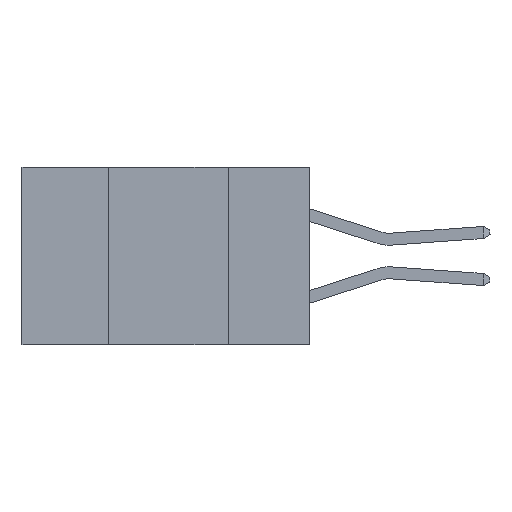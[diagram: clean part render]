
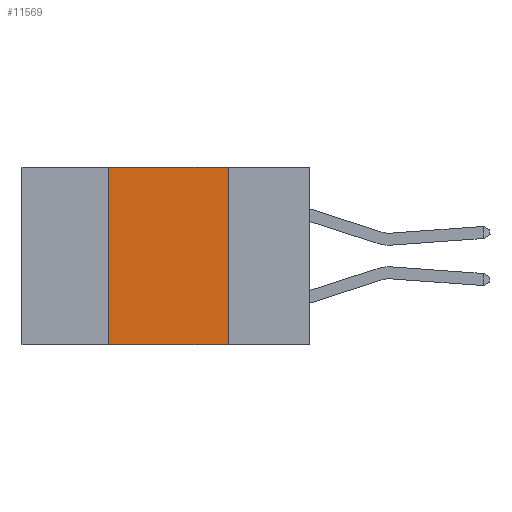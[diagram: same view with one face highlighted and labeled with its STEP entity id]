
A CAD part, left-side view. The second image highlights one B-rep face of the part: STEP entity #11569.
In plain terms, the highlighted planar face has unit normal (-1, 0, 0).
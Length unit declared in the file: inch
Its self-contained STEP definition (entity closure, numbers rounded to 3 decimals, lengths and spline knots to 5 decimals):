
#96 = ORIENTED_EDGE ( 'NONE', *, *, #4478, .F. ) ;
#165 = CARTESIAN_POINT ( 'NONE',  ( 0., 0.17, -0.37 ) ) ;
#1410 = LINE ( 'NONE', #9812, #3925 ) ;
#1760 = PLANE ( 'NONE',  #5299 ) ;
#1790 = VERTEX_POINT ( 'NONE', #10025 ) ;
#1830 = VECTOR ( 'NONE', #5807, 39.37008 ) ;
#1998 = VECTOR ( 'NONE', #4854, 39.37008 ) ;
#2380 = VERTEX_POINT ( 'NONE', #11120 ) ;
#3196 = EDGE_CURVE ( 'NONE', #1790, #10162, #1410, .T. ) ;
#3392 = ORIENTED_EDGE ( 'NONE', *, *, #6930, .F. ) ;
#3659 = DIRECTION ( 'NONE',  ( 1., 0., 0. ) ) ;
#3826 = EDGE_CURVE ( 'NONE', #1790, #2380, #4532, .T. ) ;
#3925 = VECTOR ( 'NONE', #9956, 39.37008 ) ;
#4478 = EDGE_CURVE ( 'NONE', #2380, #6053, #4930, .T. ) ;
#4532 = LINE ( 'NONE', #4841, #1998 ) ;
#4841 = CARTESIAN_POINT ( 'NONE',  ( 0., 0.42, -0.37 ) ) ;
#4854 = DIRECTION ( 'NONE',  ( 0., 0., 1. ) ) ;
#4930 = LINE ( 'NONE', #6743, #1830 ) ;
#5299 = AXIS2_PLACEMENT_3D ( 'NONE', #6426, #3659, #10152 ) ;
#5807 = DIRECTION ( 'NONE',  ( 0., -1., 0. ) ) ;
#6053 = VERTEX_POINT ( 'NONE', #11933 ) ;
#6426 = CARTESIAN_POINT ( 'NONE',  ( 0., 0.6, 0. ) ) ;
#6636 = FACE_OUTER_BOUND ( 'NONE', #7330, .T. ) ;
#6743 = CARTESIAN_POINT ( 'NONE',  ( 0., 0.6, 0. ) ) ;
#6930 = EDGE_CURVE ( 'NONE', #6053, #10162, #9798, .T. ) ;
#7330 = EDGE_LOOP ( 'NONE', ( #3392, #96, #8150, #9254 ) ) ;
#7567 = DIRECTION ( 'NONE',  ( 0., 0., -1. ) ) ;
#8150 = ORIENTED_EDGE ( 'NONE', *, *, #3826, .F. ) ;
#8582 = CARTESIAN_POINT ( 'NONE',  ( 0., 0.17, -0.37 ) ) ;
#9254 = ORIENTED_EDGE ( 'NONE', *, *, #3196, .T. ) ;
#9798 = LINE ( 'NONE', #165, #11911 ) ;
#9812 = CARTESIAN_POINT ( 'NONE',  ( 0., 0.6, -0.37 ) ) ;
#9956 = DIRECTION ( 'NONE',  ( 0., -1., 0. ) ) ;
#10025 = CARTESIAN_POINT ( 'NONE',  ( 0., 0.42, -0.37 ) ) ;
#10152 = DIRECTION ( 'NONE',  ( 0., 0., -1. ) ) ;
#10162 = VERTEX_POINT ( 'NONE', #8582 ) ;
#11120 = CARTESIAN_POINT ( 'NONE',  ( 0., 0.42, 0. ) ) ;
#11569 = ADVANCED_FACE ( 'NONE', ( #6636 ), #1760, .F. ) ;
#11911 = VECTOR ( 'NONE', #7567, 39.37008 ) ;
#11933 = CARTESIAN_POINT ( 'NONE',  ( 0., 0.17, 0. ) ) ;
